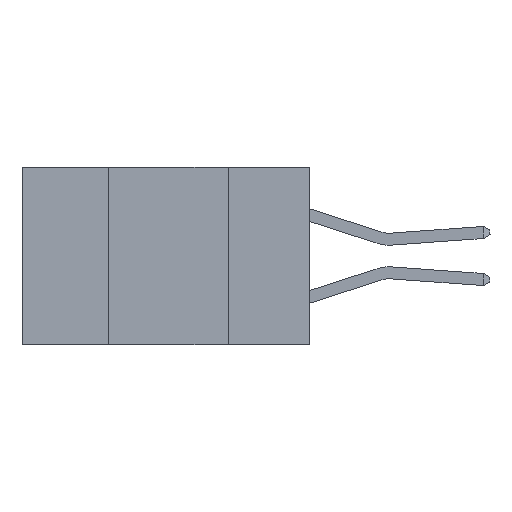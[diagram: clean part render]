
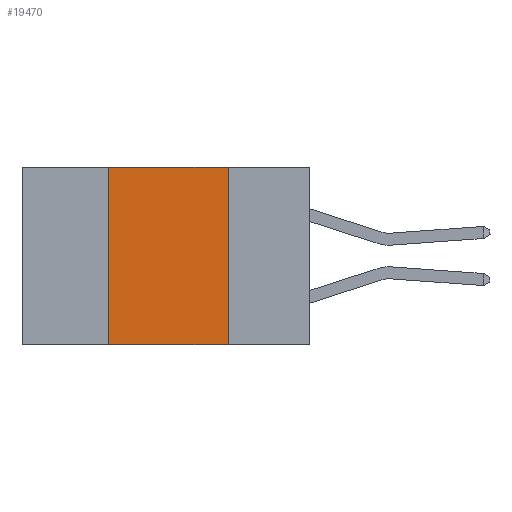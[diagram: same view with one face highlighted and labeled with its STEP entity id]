
A CAD part, left-side view. The second image highlights one B-rep face of the part: STEP entity #19470.
In plain terms, the highlighted planar face has unit normal (-1, 0, 0).
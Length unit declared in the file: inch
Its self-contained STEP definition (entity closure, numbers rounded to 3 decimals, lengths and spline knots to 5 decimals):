
#673 = ORIENTED_EDGE ( 'NONE', *, *, #13976, .F. ) ;
#1469 = VECTOR ( 'NONE', #12307, 39.37008 ) ;
#1744 = VECTOR ( 'NONE', #14834, 39.37008 ) ;
#1944 = VERTEX_POINT ( 'NONE', #20994 ) ;
#2807 = ORIENTED_EDGE ( 'NONE', *, *, #8240, .F. ) ;
#3126 = DIRECTION ( 'NONE',  ( 1., 0., 0. ) ) ;
#3841 = EDGE_CURVE ( 'NONE', #5088, #11473, #18028, .T. ) ;
#4164 = DIRECTION ( 'NONE',  ( 0., 0., 1. ) ) ;
#4183 = EDGE_CURVE ( 'NONE', #5088, #9891, #17323, .T. ) ;
#4640 = CARTESIAN_POINT ( 'NONE',  ( 0., 0.6, 0. ) ) ;
#5088 = VERTEX_POINT ( 'NONE', #10513 ) ;
#6251 = LINE ( 'NONE', #9685, #1744 ) ;
#6365 = PLANE ( 'NONE',  #13687 ) ;
#8240 = EDGE_CURVE ( 'NONE', #1944, #9891, #16816, .T. ) ;
#8903 = VECTOR ( 'NONE', #4164, 39.37008 ) ;
#9336 = CARTESIAN_POINT ( 'NONE',  ( 0., 0.42, -0.37 ) ) ;
#9685 = CARTESIAN_POINT ( 'NONE',  ( 0., 0.6, 0. ) ) ;
#9891 = VERTEX_POINT ( 'NONE', #17598 ) ;
#10375 = VECTOR ( 'NONE', #20134, 39.37008 ) ;
#10513 = CARTESIAN_POINT ( 'NONE',  ( 0., 0.42, -0.37 ) ) ;
#11094 = CARTESIAN_POINT ( 'NONE',  ( 0., 0.17, -0.37 ) ) ;
#11473 = VERTEX_POINT ( 'NONE', #21032 ) ;
#11975 = FACE_OUTER_BOUND ( 'NONE', #15704, .T. ) ;
#12307 = DIRECTION ( 'NONE',  ( 0., -1., 0. ) ) ;
#13677 = DIRECTION ( 'NONE',  ( 0., 0., -1. ) ) ;
#13687 = AXIS2_PLACEMENT_3D ( 'NONE', #4640, #3126, #13677 ) ;
#13976 = EDGE_CURVE ( 'NONE', #11473, #1944, #6251, .T. ) ;
#14770 = ORIENTED_EDGE ( 'NONE', *, *, #4183, .T. ) ;
#14834 = DIRECTION ( 'NONE',  ( 0., -1., 0. ) ) ;
#15704 = EDGE_LOOP ( 'NONE', ( #2807, #673, #15958, #14770 ) ) ;
#15958 = ORIENTED_EDGE ( 'NONE', *, *, #3841, .F. ) ;
#16816 = LINE ( 'NONE', #11094, #10375 ) ;
#17323 = LINE ( 'NONE', #21097, #1469 ) ;
#17598 = CARTESIAN_POINT ( 'NONE',  ( 0., 0.17, -0.37 ) ) ;
#18028 = LINE ( 'NONE', #9336, #8903 ) ;
#19470 = ADVANCED_FACE ( 'NONE', ( #11975 ), #6365, .F. ) ;
#20134 = DIRECTION ( 'NONE',  ( 0., 0., -1. ) ) ;
#20994 = CARTESIAN_POINT ( 'NONE',  ( 0., 0.17, 0. ) ) ;
#21032 = CARTESIAN_POINT ( 'NONE',  ( 0., 0.42, 0. ) ) ;
#21097 = CARTESIAN_POINT ( 'NONE',  ( 0., 0.6, -0.37 ) ) ;
